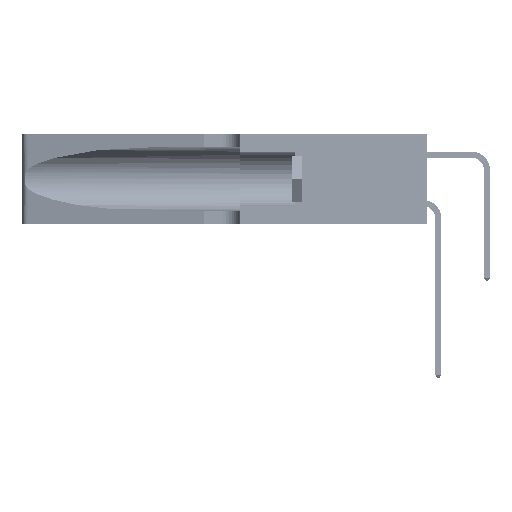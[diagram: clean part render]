
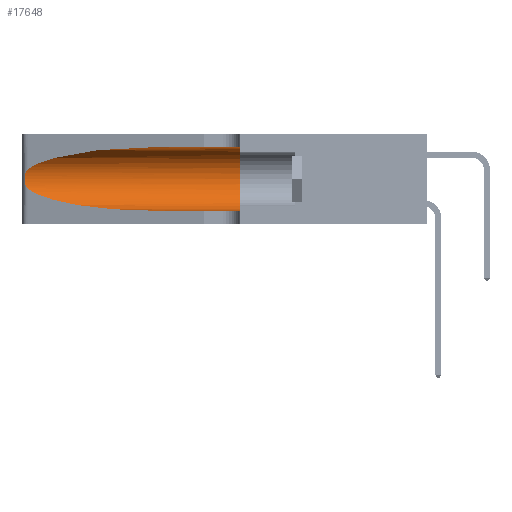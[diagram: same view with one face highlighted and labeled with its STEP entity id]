
A CAD part, left-side view. The second image highlights one B-rep face of the part: STEP entity #17648.
In plain terms, the highlighted cylindrical face has radius 3.308 mm (diameter 6.617 mm), a partial arc.
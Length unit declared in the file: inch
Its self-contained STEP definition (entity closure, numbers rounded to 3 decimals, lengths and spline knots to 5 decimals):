
#196 = CARTESIAN_POINT ( 'NONE',  ( 0.1305, 0.72297, 0.05475 ) ) ;
#897 = CARTESIAN_POINT ( 'NONE',  ( 0.25854, 1.2359, 0.20912 ) ) ;
#1240 = ORIENTED_EDGE ( 'NONE', *, *, #2690, .T. ) ;
#1890 = CARTESIAN_POINT ( 'NONE',  ( 0.25487, 1.22718, 0.14631 ) ) ;
#1967 = EDGE_CURVE ( 'NONE', #21082, #28800, #3982, .T. ) ;
#2690 = EDGE_CURVE ( 'NONE', #52483, #21082, #11864, .T. ) ;
#3957 = EDGE_CURVE ( 'NONE', #41427, #10746, #42129, .T. ) ;
#3982 =( BOUNDED_CURVE ( )  B_SPLINE_CURVE ( 3, ( #21394, #46553, #50816, #25636 ),
 .UNSPECIFIED., .F., .T. ) 
 B_SPLINE_CURVE_WITH_KNOTS ( ( 4, 4 ),
 ( 3.44316, 4.71239 ),
 .UNSPECIFIED. ) 
 CURVE ( )  GEOMETRIC_REPRESENTATION_ITEM ( )  RATIONAL_B_SPLINE_CURVE ( ( 1., 0.87, 0.87, 1. ) ) 
 REPRESENTATION_ITEM ( '' )  );
#4642 = CARTESIAN_POINT ( 'NONE',  ( 0.1305, 0.35, 0.185 ) ) ;
#4936 = CARTESIAN_POINT ( 'NONE',  ( 0.25555, 1.22994, 0.2215 ) ) ;
#5119 = CARTESIAN_POINT ( 'NONE',  ( 0.26075, 1.23896, 0.19203 ) ) ;
#7515 = ORIENTED_EDGE ( 'NONE', *, *, #21597, .F. ) ;
#8881 = DIRECTION ( 'NONE',  ( 0., 0., 1. ) ) ;
#9321 = CARTESIAN_POINT ( 'NONE',  ( 0.25487, 1.22718, 0.22369 ) ) ;
#9359 = CARTESIAN_POINT ( 'NONE',  ( 0.26017, 1.23833, 0.17102 ) ) ;
#10746 = VERTEX_POINT ( 'NONE', #36131 ) ;
#11864 = B_SPLINE_CURVE_WITH_KNOTS ( 'NONE', 3,
 ( #34384, #4936, #51285, #26103, #897, #30336, #5119, #34562, #9359, #38807, #13570, #43024, #17843, #47221 ),
 .UNSPECIFIED., .F., .F.,
 ( 4, 2, 2, 2, 2, 2, 4 ),
 ( 0., 0.00027, 0.00053, 0.00107, 0.0016, 0.00187, 0.00214 ),
 .UNSPECIFIED. ) ;
#12573 = CYLINDRICAL_SURFACE ( 'NONE', #52106, 0.13025 ) ;
#13170 = DIRECTION ( 'NONE',  ( 0., -1., 0. ) ) ;
#13403 = CARTESIAN_POINT ( 'NONE',  ( 0.1305, 1.61858, 0.31525 ) ) ;
#13570 = CARTESIAN_POINT ( 'NONE',  ( 0.25789, 1.23486, 0.15765 ) ) ;
#16004 = CARTESIAN_POINT ( 'NONE',  ( 0.1305, 0.72297, 0.31525 ) ) ;
#17648 = ADVANCED_FACE ( 'NONE', ( #46124 ), #12573, .F. ) ;
#17843 = CARTESIAN_POINT ( 'NONE',  ( 0.25555, 1.22993, 0.14849 ) ) ;
#21082 = VERTEX_POINT ( 'NONE', #1890 ) ;
#21394 = CARTESIAN_POINT ( 'NONE',  ( 0.25487, 1.22718, 0.14631 ) ) ;
#21597 = EDGE_CURVE ( 'NONE', #40730, #41427, #46715, .T. ) ;
#21912 = VECTOR ( 'NONE', #13170, 39.37008 ) ;
#24539 = LINE ( 'NONE', #46644, #21912 ) ;
#25636 = CARTESIAN_POINT ( 'NONE',  ( 0.1305, 0.72297, 0.05475 ) ) ;
#26103 = CARTESIAN_POINT ( 'NONE',  ( 0.25787, 1.23484, 0.2124 ) ) ;
#28705 = CARTESIAN_POINT ( 'NONE',  ( 0.25487, 1.22718, 0.22369 ) ) ;
#28800 = VERTEX_POINT ( 'NONE', #196 ) ;
#29534 = ORIENTED_EDGE ( 'NONE', *, *, #3957, .F. ) ;
#29586 = EDGE_CURVE ( 'NONE', #28800, #10746, #24539, .T. ) ;
#30171 = DIRECTION ( 'NONE',  ( 0., -1., 0. ) ) ;
#30336 = CARTESIAN_POINT ( 'NONE',  ( 0.26018, 1.23835, 0.19895 ) ) ;
#34074 = DIRECTION ( 'NONE',  ( 0., 1., 0. ) ) ;
#34384 = CARTESIAN_POINT ( 'NONE',  ( 0.25487, 1.22718, 0.22369 ) ) ;
#34562 = CARTESIAN_POINT ( 'NONE',  ( 0.26075, 1.23896, 0.178 ) ) ;
#36131 = CARTESIAN_POINT ( 'NONE',  ( 0.1305, 0.35, 0.05475 ) ) ;
#37285 = CARTESIAN_POINT ( 'NONE',  ( 0.1305, 0.72297, 0.31525 ) ) ;
#38228 = VECTOR ( 'NONE', #30171, 39.37008 ) ;
#38319 = DIRECTION ( 'NONE',  ( 0., 0., -1. ) ) ;
#38807 = CARTESIAN_POINT ( 'NONE',  ( 0.25856, 1.23593, 0.16098 ) ) ;
#40730 = VERTEX_POINT ( 'NONE', #37285 ) ;
#41210 = CARTESIAN_POINT ( 'NONE',  ( 0.18966, 0.96281, 0.31525 ) ) ;
#41426 = CARTESIAN_POINT ( 'NONE',  ( 0.1305, 0.35, 0.31525 ) ) ;
#41427 = VERTEX_POINT ( 'NONE', #41426 ) ;
#42129 = CIRCLE ( 'NONE', #46056, 0.13025 ) ;
#43024 = CARTESIAN_POINT ( 'NONE',  ( 0.25639, 1.23186, 0.15144 ) ) ;
#43092 = ORIENTED_EDGE ( 'NONE', *, *, #50446, .T. ) ;
#43214 =( BOUNDED_CURVE ( )  B_SPLINE_CURVE ( 3, ( #16004, #41210, #53878, #28705 ),
 .UNSPECIFIED., .F., .F. ) 
 B_SPLINE_CURVE_WITH_KNOTS ( ( 4, 4 ),
 ( 1.5708, 2.84003 ),
 .UNSPECIFIED. ) 
 CURVE ( )  GEOMETRIC_REPRESENTATION_ITEM ( )  RATIONAL_B_SPLINE_CURVE ( ( 1., 0.87, 0.87, 1. ) ) 
 REPRESENTATION_ITEM ( '' )  );
#46056 = AXIS2_PLACEMENT_3D ( 'NONE', #4642, #34074, #8881 ) ;
#46124 = FACE_OUTER_BOUND ( 'NONE', #51887, .T. ) ;
#46553 = CARTESIAN_POINT ( 'NONE',  ( 0.2373, 1.15595, 0.08982 ) ) ;
#46644 = CARTESIAN_POINT ( 'NONE',  ( 0.1305, 1.61858, 0.05475 ) ) ;
#46715 = LINE ( 'NONE', #13403, #38228 ) ;
#46720 = CARTESIAN_POINT ( 'NONE',  ( 0.1305, 1.61858, 0.185 ) ) ;
#47221 = CARTESIAN_POINT ( 'NONE',  ( 0.25487, 1.22718, 0.14631 ) ) ;
#48855 = ORIENTED_EDGE ( 'NONE', *, *, #1967, .T. ) ;
#50446 = EDGE_CURVE ( 'NONE', #40730, #52483, #43214, .T. ) ;
#50816 = CARTESIAN_POINT ( 'NONE',  ( 0.18966, 0.96281, 0.05475 ) ) ;
#50969 = DIRECTION ( 'NONE',  ( 0., -1., 0. ) ) ;
#51149 = ORIENTED_EDGE ( 'NONE', *, *, #29586, .T. ) ;
#51285 = CARTESIAN_POINT ( 'NONE',  ( 0.25639, 1.23184, 0.21858 ) ) ;
#51887 = EDGE_LOOP ( 'NONE', ( #43092, #1240, #48855, #51149, #29534, #7515 ) ) ;
#52106 = AXIS2_PLACEMENT_3D ( 'NONE', #46720, #50969, #38319 ) ;
#52483 = VERTEX_POINT ( 'NONE', #9321 ) ;
#53878 = CARTESIAN_POINT ( 'NONE',  ( 0.2373, 1.15595, 0.28018 ) ) ;
